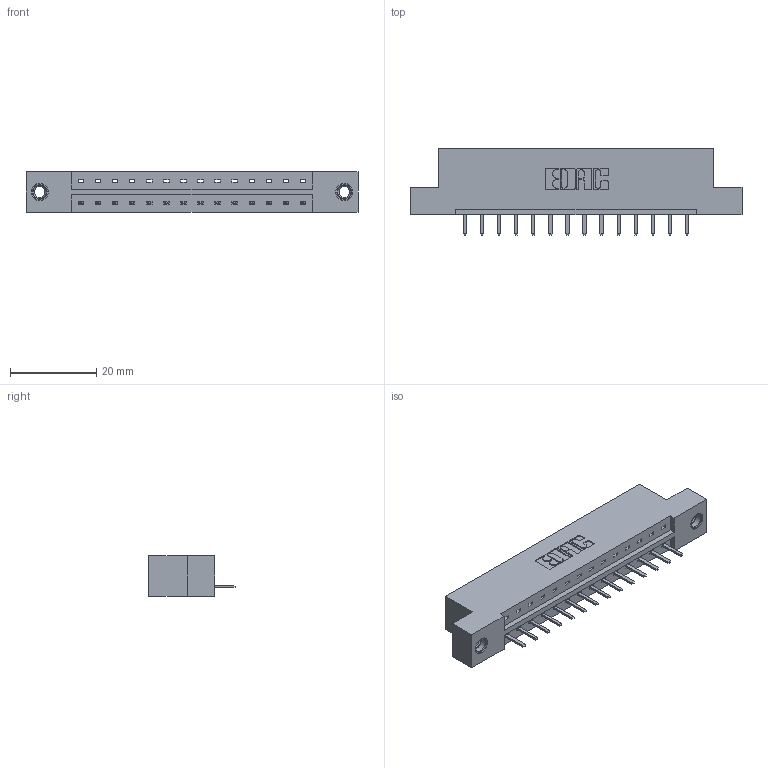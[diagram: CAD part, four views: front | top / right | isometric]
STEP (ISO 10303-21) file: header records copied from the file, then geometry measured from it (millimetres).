
FILE_DESCRIPTION (( 'STEP AP203' ), '1' );
FILE_NAME ('833-014-520-107.STEP', '2020-05-31T00:58:38', ( '' ), ( '' ), 'SwSTEP 2.0', 'SolidWorks 2020', '' );
FILE_SCHEMA (( 'CONFIG_CONTROL_DESIGN' ));
Length unit declared in the file: inch
Products named in the file (4): 833 Part_Flush - .156 Dia - TI; 345-250-001_345-250-005-103; 833-014-520-107; 345-292-001_345-293-120
Assembly tree (17 placements, depth 2):
  833-014-520-107
    833 Part_Flush - .156 Dia - TI
    345-292-001_345-293-120  x14
    345-250-001_345-250-005-103  x2
Bounding box: 77.01 x 20.02 x 9.4 mm (x, y, z)
Volume: 7455.1 mm3; surface area: 7779.2 mm2
Topology: 17 solids, 17 shells, 1042 faces, 3023 edges, 1970 vertices
Faces by surface type: plane 718, cylinder 308, cone 12, torus 4
Entity records: 13480 total; most frequent: CARTESIAN_POINT 2323, ORIENTED_EDGE 2254, DIRECTION 2037, EDGE_CURVE 1127, VECTOR 975, LINE 975, VERTEX_POINT 744, AXIS2_PLACEMENT_3D 531
